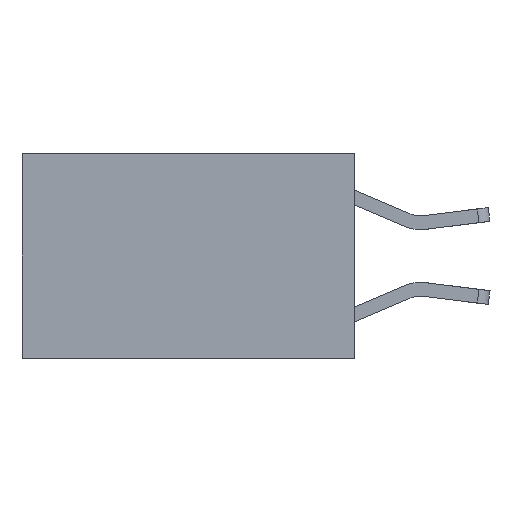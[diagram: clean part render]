
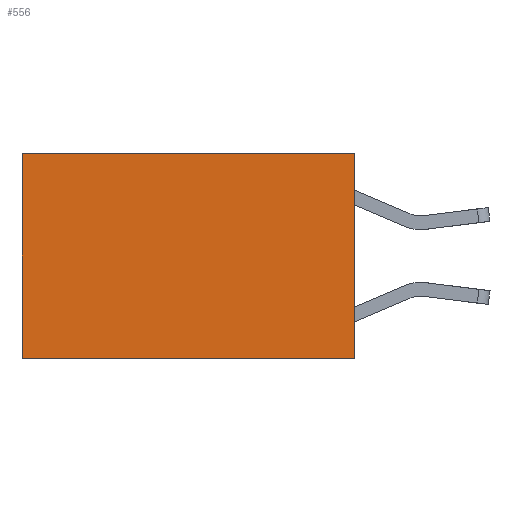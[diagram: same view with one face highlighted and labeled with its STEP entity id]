
A CAD part, left-side view. The second image highlights one B-rep face of the part: STEP entity #556.
In plain terms, the highlighted planar face has unit normal (-1, 0, 0).
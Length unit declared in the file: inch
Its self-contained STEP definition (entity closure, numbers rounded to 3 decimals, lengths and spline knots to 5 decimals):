
#319 = CARTESIAN_POINT ( 'NONE',  ( 0.2625, 0., 0. ) ) ;
#556 = ADVANCED_FACE ( 'NONE', ( #975 ), #2249, .F. ) ;
#619 = LINE ( 'NONE', #8856, #1240 ) ;
#628 = VERTEX_POINT ( 'NONE', #4569 ) ;
#975 = FACE_OUTER_BOUND ( 'NONE', #12936, .T. ) ;
#1102 = AXIS2_PLACEMENT_3D ( 'NONE', #319, #11270, #6375 ) ;
#1240 = VECTOR ( 'NONE', #9714, 39.37008 ) ;
#2224 = VERTEX_POINT ( 'NONE', #4789 ) ;
#2249 = PLANE ( 'NONE',  #1102 ) ;
#2613 = ORIENTED_EDGE ( 'NONE', *, *, #5780, .F. ) ;
#3142 = CARTESIAN_POINT ( 'NONE',  ( 0.2625, 0., 0. ) ) ;
#4518 = DIRECTION ( 'NONE',  ( 0., 1., 0. ) ) ;
#4553 = DIRECTION ( 'NONE',  ( 0., 0., -1. ) ) ;
#4569 = CARTESIAN_POINT ( 'NONE',  ( 0.2625, 0., -0.37 ) ) ;
#4783 = DIRECTION ( 'NONE',  ( 0., 1., 0. ) ) ;
#4789 = CARTESIAN_POINT ( 'NONE',  ( 0.2625, 0.6, 0. ) ) ;
#5630 = VECTOR ( 'NONE', #4783, 39.37008 ) ;
#5780 = EDGE_CURVE ( 'NONE', #628, #9744, #7847, .T. ) ;
#6295 = CARTESIAN_POINT ( 'NONE',  ( 0.2625, 0., 0. ) ) ;
#6375 = DIRECTION ( 'NONE',  ( 0., 0., -1. ) ) ;
#6494 = EDGE_CURVE ( 'NONE', #2224, #9744, #619, .T. ) ;
#7310 = VERTEX_POINT ( 'NONE', #3142 ) ;
#7555 = VECTOR ( 'NONE', #4518, 39.37008 ) ;
#7847 = LINE ( 'NONE', #10877, #5630 ) ;
#8856 = CARTESIAN_POINT ( 'NONE',  ( 0.2625, 0.6, 0. ) ) ;
#8873 = CARTESIAN_POINT ( 'NONE',  ( 0.2625, 0.6, -0.37 ) ) ;
#9153 = LINE ( 'NONE', #9524, #7555 ) ;
#9446 = VECTOR ( 'NONE', #4553, 39.37008 ) ;
#9466 = ORIENTED_EDGE ( 'NONE', *, *, #6494, .T. ) ;
#9524 = CARTESIAN_POINT ( 'NONE',  ( 0.2625, 0., 0. ) ) ;
#9714 = DIRECTION ( 'NONE',  ( 0., 0., -1. ) ) ;
#9744 = VERTEX_POINT ( 'NONE', #8873 ) ;
#10733 = EDGE_CURVE ( 'NONE', #7310, #2224, #9153, .T. ) ;
#10877 = CARTESIAN_POINT ( 'NONE',  ( 0.2625, 0., -0.37 ) ) ;
#11119 = ORIENTED_EDGE ( 'NONE', *, *, #10733, .T. ) ;
#11254 = EDGE_CURVE ( 'NONE', #7310, #628, #12094, .T. ) ;
#11270 = DIRECTION ( 'NONE',  ( 1., 0., 0. ) ) ;
#12094 = LINE ( 'NONE', #6295, #9446 ) ;
#12408 = ORIENTED_EDGE ( 'NONE', *, *, #11254, .F. ) ;
#12936 = EDGE_LOOP ( 'NONE', ( #9466, #2613, #12408, #11119 ) ) ;
